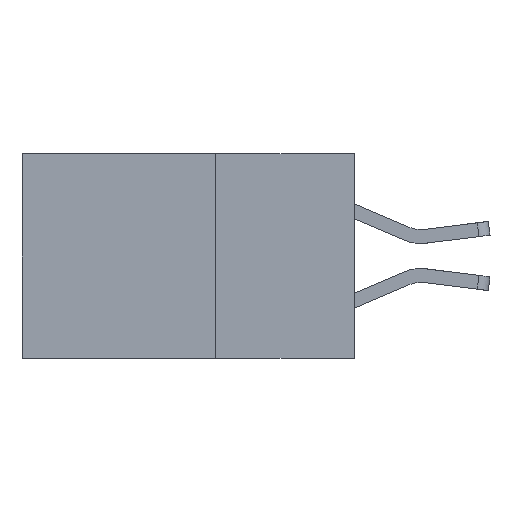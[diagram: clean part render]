
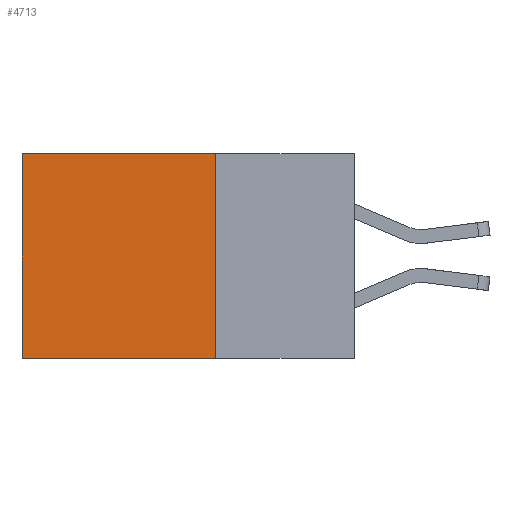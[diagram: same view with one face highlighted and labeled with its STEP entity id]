
A CAD part, left-side view. The second image highlights one B-rep face of the part: STEP entity #4713.
In plain terms, the highlighted planar face has unit normal (-1, 0, 0).
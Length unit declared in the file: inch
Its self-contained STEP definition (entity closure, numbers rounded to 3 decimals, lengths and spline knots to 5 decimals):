
#134 = CARTESIAN_POINT ( 'NONE',  ( 0.2615, 0.25, -0.37 ) ) ;
#493 = EDGE_CURVE ( 'NONE', #2797, #1741, #2715, .T. ) ;
#505 = ORIENTED_EDGE ( 'NONE', *, *, #493, .T. ) ;
#1026 = CARTESIAN_POINT ( 'NONE',  ( 0.2615, 0.6, -0.37 ) ) ;
#1567 = CARTESIAN_POINT ( 'NONE',  ( 0.2615, 0.25, -0.37 ) ) ;
#1616 = DIRECTION ( 'NONE',  ( 0., 0., -1. ) ) ;
#1741 = VERTEX_POINT ( 'NONE', #3497 ) ;
#1768 = ORIENTED_EDGE ( 'NONE', *, *, #6814, .F. ) ;
#1799 = LINE ( 'NONE', #7270, #7980 ) ;
#1905 = CARTESIAN_POINT ( 'NONE',  ( 0.2615, 0.25, -0.37 ) ) ;
#2100 = EDGE_CURVE ( 'NONE', #8457, #4305, #7278, .T. ) ;
#2467 = DIRECTION ( 'NONE',  ( 0., 0., -1. ) ) ;
#2715 = LINE ( 'NONE', #6713, #6161 ) ;
#2797 = VERTEX_POINT ( 'NONE', #9055 ) ;
#2860 = DIRECTION ( 'NONE',  ( 0., 1., 0. ) ) ;
#3497 = CARTESIAN_POINT ( 'NONE',  ( 0.2615, 0.6, 0. ) ) ;
#3777 = EDGE_CURVE ( 'NONE', #1741, #4305, #1799, .T. ) ;
#4305 = VERTEX_POINT ( 'NONE', #1026 ) ;
#4649 = DIRECTION ( 'NONE',  ( 1., 0., 0. ) ) ;
#4713 = ADVANCED_FACE ( 'NONE', ( #5461 ), #9289, .F. ) ;
#5107 = VECTOR ( 'NONE', #2467, 39.37008 ) ;
#5461 = FACE_OUTER_BOUND ( 'NONE', #8622, .T. ) ;
#6161 = VECTOR ( 'NONE', #2860, 39.37008 ) ;
#6638 = VECTOR ( 'NONE', #8811, 39.37008 ) ;
#6713 = CARTESIAN_POINT ( 'NONE',  ( 0.2615, 0.25, 0. ) ) ;
#6814 = EDGE_CURVE ( 'NONE', #2797, #8457, #7281, .T. ) ;
#7270 = CARTESIAN_POINT ( 'NONE',  ( 0.2615, 0.6, -0.37 ) ) ;
#7278 = LINE ( 'NONE', #1905, #6638 ) ;
#7281 = LINE ( 'NONE', #134, #5107 ) ;
#7346 = ORIENTED_EDGE ( 'NONE', *, *, #3777, .T. ) ;
#7980 = VECTOR ( 'NONE', #8902, 39.37008 ) ;
#8192 = ORIENTED_EDGE ( 'NONE', *, *, #2100, .F. ) ;
#8320 = AXIS2_PLACEMENT_3D ( 'NONE', #1567, #4649, #1616 ) ;
#8405 = CARTESIAN_POINT ( 'NONE',  ( 0.2615, 0.25, -0.37 ) ) ;
#8457 = VERTEX_POINT ( 'NONE', #8405 ) ;
#8622 = EDGE_LOOP ( 'NONE', ( #7346, #8192, #1768, #505 ) ) ;
#8811 = DIRECTION ( 'NONE',  ( 0., 1., 0. ) ) ;
#8902 = DIRECTION ( 'NONE',  ( 0., 0., -1. ) ) ;
#9055 = CARTESIAN_POINT ( 'NONE',  ( 0.2615, 0.25, 0. ) ) ;
#9289 = PLANE ( 'NONE',  #8320 ) ;
